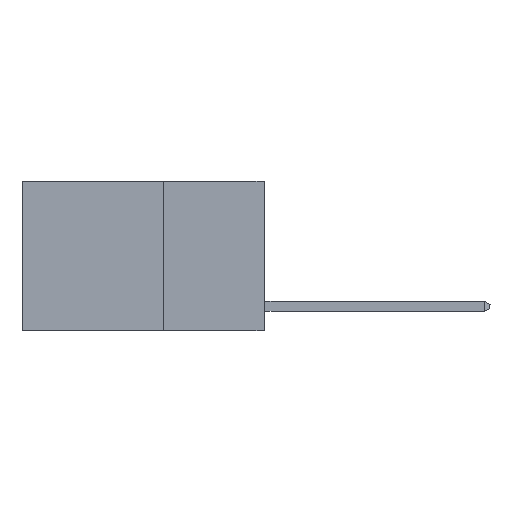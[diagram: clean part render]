
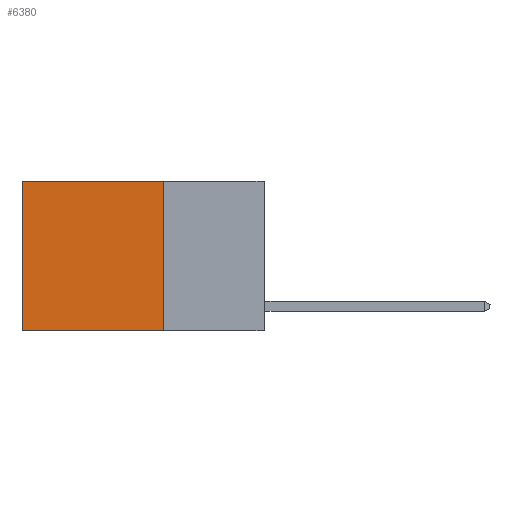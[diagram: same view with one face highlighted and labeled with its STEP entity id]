
A CAD part, left-side view. The second image highlights one B-rep face of the part: STEP entity #6380.
In plain terms, the highlighted planar face has unit normal (-1, 0, 0).
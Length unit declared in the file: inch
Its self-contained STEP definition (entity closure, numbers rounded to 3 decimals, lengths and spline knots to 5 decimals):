
#749 = VECTOR ( 'NONE', #11959, 39.37008 ) ;
#1037 = DIRECTION ( 'NONE',  ( 0., 1., 0. ) ) ;
#1777 = PLANE ( 'NONE',  #8807 ) ;
#1915 = EDGE_CURVE ( 'NONE', #11264, #5709, #6188, .T. ) ;
#2158 = CARTESIAN_POINT ( 'NONE',  ( 0.2625, 0.25, 0. ) ) ;
#2256 = EDGE_LOOP ( 'NONE', ( #11090, #2605, #7577, #11668 ) ) ;
#2605 = ORIENTED_EDGE ( 'NONE', *, *, #2947, .F. ) ;
#2843 = LINE ( 'NONE', #6801, #3761 ) ;
#2947 = EDGE_CURVE ( 'NONE', #11235, #4056, #9596, .T. ) ;
#3246 = FACE_OUTER_BOUND ( 'NONE', #2256, .T. ) ;
#3513 = EDGE_CURVE ( 'NONE', #5709, #4056, #10024, .T. ) ;
#3761 = VECTOR ( 'NONE', #7663, 39.37008 ) ;
#4056 = VERTEX_POINT ( 'NONE', #7881 ) ;
#4966 = VECTOR ( 'NONE', #1037, 39.37008 ) ;
#5697 = DIRECTION ( 'NONE',  ( 1., 0., 0. ) ) ;
#5709 = VERTEX_POINT ( 'NONE', #6694 ) ;
#5729 = CARTESIAN_POINT ( 'NONE',  ( 0.2625, 0.6, 0. ) ) ;
#6188 = LINE ( 'NONE', #2158, #749 ) ;
#6380 = ADVANCED_FACE ( 'NONE', ( #3246 ), #1777, .F. ) ;
#6694 = CARTESIAN_POINT ( 'NONE',  ( 0.2625, 0.6, 0. ) ) ;
#6801 = CARTESIAN_POINT ( 'NONE',  ( 0.2625, 0.25, 0. ) ) ;
#7445 = DIRECTION ( 'NONE',  ( 0., 0., -1. ) ) ;
#7577 = ORIENTED_EDGE ( 'NONE', *, *, #9673, .F. ) ;
#7663 = DIRECTION ( 'NONE',  ( 0., 0., -1. ) ) ;
#7827 = CARTESIAN_POINT ( 'NONE',  ( 0.2625, 0.25, -0.37 ) ) ;
#7881 = CARTESIAN_POINT ( 'NONE',  ( 0.2625, 0.6, -0.37 ) ) ;
#8579 = DIRECTION ( 'NONE',  ( 0., 0., -1. ) ) ;
#8807 = AXIS2_PLACEMENT_3D ( 'NONE', #11390, #5697, #8579 ) ;
#9596 = LINE ( 'NONE', #7827, #4966 ) ;
#9673 = EDGE_CURVE ( 'NONE', #11264, #11235, #2843, .T. ) ;
#9948 = CARTESIAN_POINT ( 'NONE',  ( 0.2625, 0.25, 0. ) ) ;
#10024 = LINE ( 'NONE', #5729, #10939 ) ;
#10227 = CARTESIAN_POINT ( 'NONE',  ( 0.2625, 0.25, -0.37 ) ) ;
#10939 = VECTOR ( 'NONE', #7445, 39.37008 ) ;
#11090 = ORIENTED_EDGE ( 'NONE', *, *, #3513, .T. ) ;
#11235 = VERTEX_POINT ( 'NONE', #10227 ) ;
#11264 = VERTEX_POINT ( 'NONE', #9948 ) ;
#11390 = CARTESIAN_POINT ( 'NONE',  ( 0.2625, 0.25, 0. ) ) ;
#11668 = ORIENTED_EDGE ( 'NONE', *, *, #1915, .T. ) ;
#11959 = DIRECTION ( 'NONE',  ( 0., 1., 0. ) ) ;
